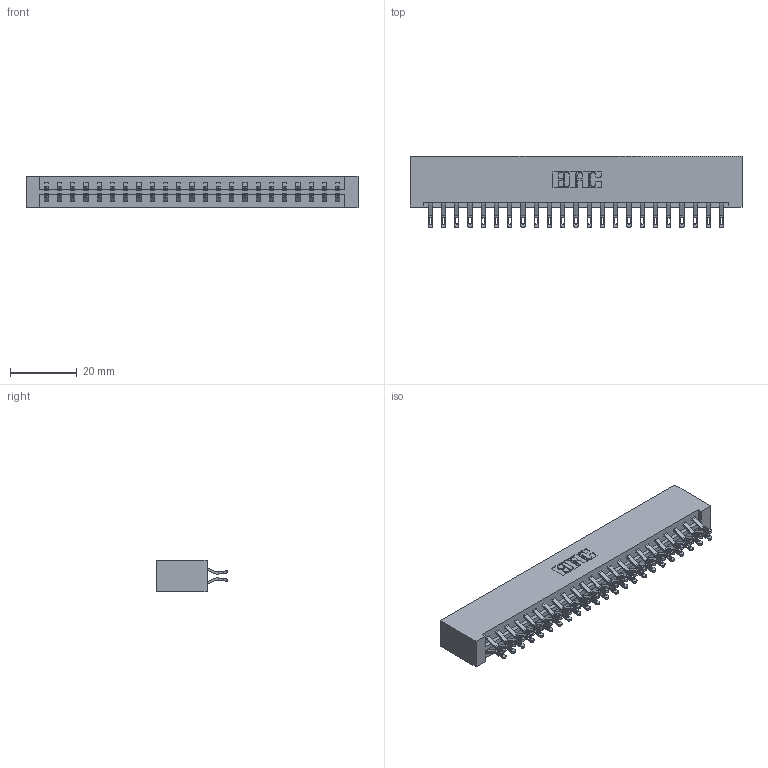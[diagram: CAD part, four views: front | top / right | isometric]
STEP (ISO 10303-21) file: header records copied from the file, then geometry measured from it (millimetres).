
FILE_DESCRIPTION (( 'STEP AP203' ), '1' );
FILE_NAME ('833-046-555-201.STEP', '2020-06-04T14:43:25', ( '' ), ( '' ), 'SwSTEP 2.0', 'SolidWorks 2020', '' );
FILE_SCHEMA (( 'CONFIG_CONTROL_DESIGN' ));
Length unit declared in the file: inch
Products named in the file (3): 833 Part_Lugless; 345-292-001_555 Tail; 833-046-555-201
Assembly tree (47 placements, depth 2):
  833-046-555-201
    833 Part_Lugless
    345-292-001_555 Tail  x46
Bounding box: 99.39 x 21.47 x 9.4 mm (x, y, z)
Volume: 10735.1 mm3; surface area: 13010.8 mm2
Topology: 47 solids, 47 shells, 2774 faces, 8705 edges, 5802 vertices
Faces by surface type: plane 1630, cylinder 1144
Entity records: 17303 total; most frequent: CARTESIAN_POINT 2924, ORIENTED_EDGE 2830, DIRECTION 2495, EDGE_CURVE 1415, LINE 1275, VECTOR 1275, VERTEX_POINT 942, AXIS2_PLACEMENT_3D 610
